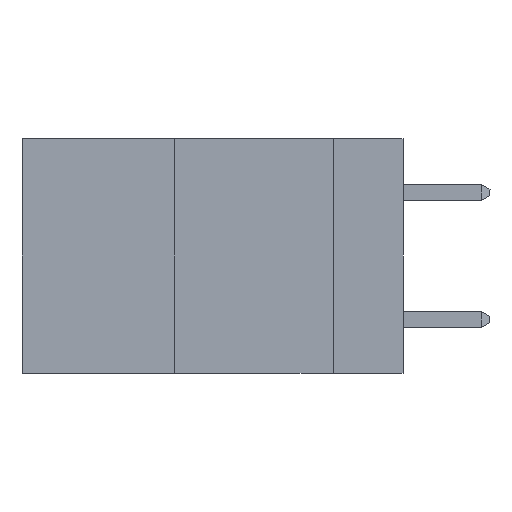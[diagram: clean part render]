
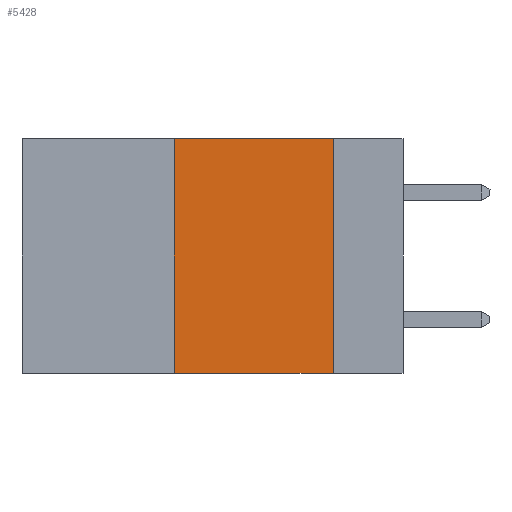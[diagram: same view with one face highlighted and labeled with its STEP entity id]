
A CAD part, left-side view. The second image highlights one B-rep face of the part: STEP entity #5428.
In plain terms, the highlighted planar face has unit normal (-1, 0, 0).
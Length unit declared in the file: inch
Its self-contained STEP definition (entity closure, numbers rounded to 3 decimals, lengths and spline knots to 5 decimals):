
#205 = CARTESIAN_POINT ( 'NONE',  ( 0., 0.36, 0. ) ) ;
#417 = VERTEX_POINT ( 'NONE', #2722 ) ;
#520 = VECTOR ( 'NONE', #8172, 39.37008 ) ;
#575 = EDGE_CURVE ( 'NONE', #417, #3092, #7211, .T. ) ;
#888 = CARTESIAN_POINT ( 'NONE',  ( 0., 0.36, -0.37 ) ) ;
#1705 = VECTOR ( 'NONE', #3215, 39.37008 ) ;
#1771 = CARTESIAN_POINT ( 'NONE',  ( 0., 0.11, 0. ) ) ;
#2099 = EDGE_CURVE ( 'NONE', #9018, #417, #4746, .T. ) ;
#2722 = CARTESIAN_POINT ( 'NONE',  ( 0., 0.36, 0. ) ) ;
#3019 = EDGE_LOOP ( 'NONE', ( #8596, #8793, #5387, #7436 ) ) ;
#3092 = VERTEX_POINT ( 'NONE', #1771 ) ;
#3149 = DIRECTION ( 'NONE',  ( 0., 0., -1. ) ) ;
#3215 = DIRECTION ( 'NONE',  ( 0., -1., 0. ) ) ;
#3335 = DIRECTION ( 'NONE',  ( 0., 0., -1. ) ) ;
#3928 = CARTESIAN_POINT ( 'NONE',  ( 0., 0.6, 0. ) ) ;
#3939 = DIRECTION ( 'NONE',  ( 1., 0., 0. ) ) ;
#4075 = FACE_OUTER_BOUND ( 'NONE', #3019, .T. ) ;
#4694 = EDGE_CURVE ( 'NONE', #3092, #8624, #7647, .T. ) ;
#4746 = LINE ( 'NONE', #205, #520 ) ;
#4832 = DIRECTION ( 'NONE',  ( 0., -1., 0. ) ) ;
#4842 = CARTESIAN_POINT ( 'NONE',  ( 0., 0.6, -0.37 ) ) ;
#5387 = ORIENTED_EDGE ( 'NONE', *, *, #2099, .F. ) ;
#5428 = ADVANCED_FACE ( 'NONE', ( #4075 ), #8618, .F. ) ;
#5669 = EDGE_CURVE ( 'NONE', #9018, #8624, #8572, .T. ) ;
#6862 = CARTESIAN_POINT ( 'NONE',  ( 0., 0.11, -0.37 ) ) ;
#7211 = LINE ( 'NONE', #8326, #1705 ) ;
#7264 = AXIS2_PLACEMENT_3D ( 'NONE', #3928, #3939, #3335 ) ;
#7434 = VECTOR ( 'NONE', #3149, 39.37008 ) ;
#7436 = ORIENTED_EDGE ( 'NONE', *, *, #5669, .T. ) ;
#7647 = LINE ( 'NONE', #8635, #7434 ) ;
#8172 = DIRECTION ( 'NONE',  ( 0., 0., 1. ) ) ;
#8326 = CARTESIAN_POINT ( 'NONE',  ( 0., 0.6, 0. ) ) ;
#8364 = VECTOR ( 'NONE', #4832, 39.37008 ) ;
#8572 = LINE ( 'NONE', #4842, #8364 ) ;
#8596 = ORIENTED_EDGE ( 'NONE', *, *, #4694, .F. ) ;
#8618 = PLANE ( 'NONE',  #7264 ) ;
#8624 = VERTEX_POINT ( 'NONE', #6862 ) ;
#8635 = CARTESIAN_POINT ( 'NONE',  ( 0., 0.11, 0. ) ) ;
#8793 = ORIENTED_EDGE ( 'NONE', *, *, #575, .F. ) ;
#9018 = VERTEX_POINT ( 'NONE', #888 ) ;
